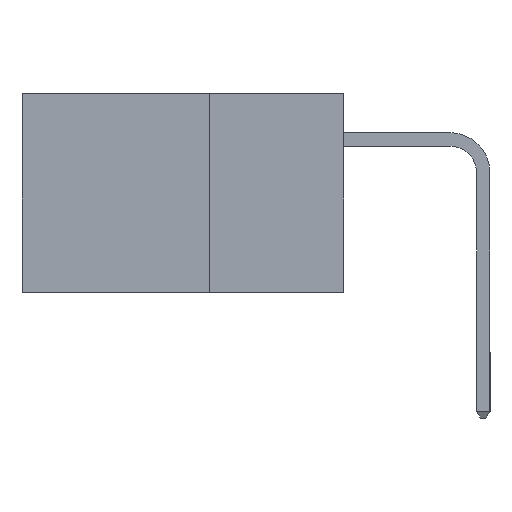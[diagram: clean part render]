
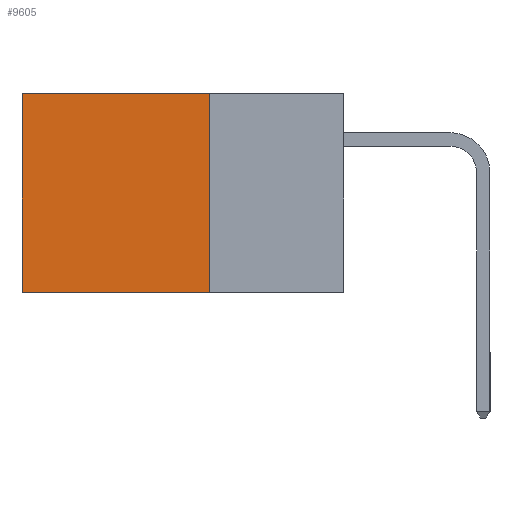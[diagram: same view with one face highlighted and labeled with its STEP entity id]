
A CAD part, left-side view. The second image highlights one B-rep face of the part: STEP entity #9605.
In plain terms, the highlighted planar face has unit normal (-1, 0, 0).
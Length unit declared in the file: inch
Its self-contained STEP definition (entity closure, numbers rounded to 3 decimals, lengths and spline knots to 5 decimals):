
#657 = CARTESIAN_POINT ( 'NONE',  ( 0.298, 0.25, 0. ) ) ;
#1942 = CARTESIAN_POINT ( 'NONE',  ( 0.298, 0.25, 0. ) ) ;
#2056 = PLANE ( 'NONE',  #4362 ) ;
#2141 = CARTESIAN_POINT ( 'NONE',  ( 0.298, 0.25, -0.37 ) ) ;
#2318 = ORIENTED_EDGE ( 'NONE', *, *, #17066, .F. ) ;
#2582 = VERTEX_POINT ( 'NONE', #17754 ) ;
#3094 = VECTOR ( 'NONE', #14684, 39.37008 ) ;
#3329 = ORIENTED_EDGE ( 'NONE', *, *, #15913, .F. ) ;
#4362 = AXIS2_PLACEMENT_3D ( 'NONE', #657, #17135, #15687 ) ;
#4766 = CARTESIAN_POINT ( 'NONE',  ( 0.298, 0.25, -0.37 ) ) ;
#6126 = EDGE_CURVE ( 'NONE', #2582, #16007, #17303, .T. ) ;
#6348 = EDGE_CURVE ( 'NONE', #10750, #2582, #17505, .T. ) ;
#6649 = ORIENTED_EDGE ( 'NONE', *, *, #6126, .T. ) ;
#6829 = DIRECTION ( 'NONE',  ( 0., 0., -1. ) ) ;
#7446 = VECTOR ( 'NONE', #6829, 39.37008 ) ;
#7762 = FACE_OUTER_BOUND ( 'NONE', #16020, .T. ) ;
#7904 = CARTESIAN_POINT ( 'NONE',  ( 0.298, 0.25, 0. ) ) ;
#8518 = LINE ( 'NONE', #2141, #9175 ) ;
#9175 = VECTOR ( 'NONE', #11552, 39.37008 ) ;
#9543 = CARTESIAN_POINT ( 'NONE',  ( 0.298, 0.6, 0. ) ) ;
#9605 = ADVANCED_FACE ( 'NONE', ( #7762 ), #2056, .F. ) ;
#10750 = VERTEX_POINT ( 'NONE', #7904 ) ;
#10833 = VECTOR ( 'NONE', #17071, 39.37008 ) ;
#10933 = ORIENTED_EDGE ( 'NONE', *, *, #6348, .T. ) ;
#11241 = LINE ( 'NONE', #17544, #3094 ) ;
#11552 = DIRECTION ( 'NONE',  ( 0., 1., 0. ) ) ;
#12518 = VERTEX_POINT ( 'NONE', #4766 ) ;
#14684 = DIRECTION ( 'NONE',  ( 0., 0., -1. ) ) ;
#15687 = DIRECTION ( 'NONE',  ( 0., 0., -1. ) ) ;
#15913 = EDGE_CURVE ( 'NONE', #12518, #16007, #8518, .T. ) ;
#16007 = VERTEX_POINT ( 'NONE', #16123 ) ;
#16020 = EDGE_LOOP ( 'NONE', ( #6649, #3329, #2318, #10933 ) ) ;
#16123 = CARTESIAN_POINT ( 'NONE',  ( 0.298, 0.6, -0.37 ) ) ;
#17066 = EDGE_CURVE ( 'NONE', #10750, #12518, #11241, .T. ) ;
#17071 = DIRECTION ( 'NONE',  ( 0., 1., 0. ) ) ;
#17135 = DIRECTION ( 'NONE',  ( 1., 0., 0. ) ) ;
#17303 = LINE ( 'NONE', #9543, #7446 ) ;
#17505 = LINE ( 'NONE', #1942, #10833 ) ;
#17544 = CARTESIAN_POINT ( 'NONE',  ( 0.298, 0.25, 0. ) ) ;
#17754 = CARTESIAN_POINT ( 'NONE',  ( 0.298, 0.6, 0. ) ) ;
